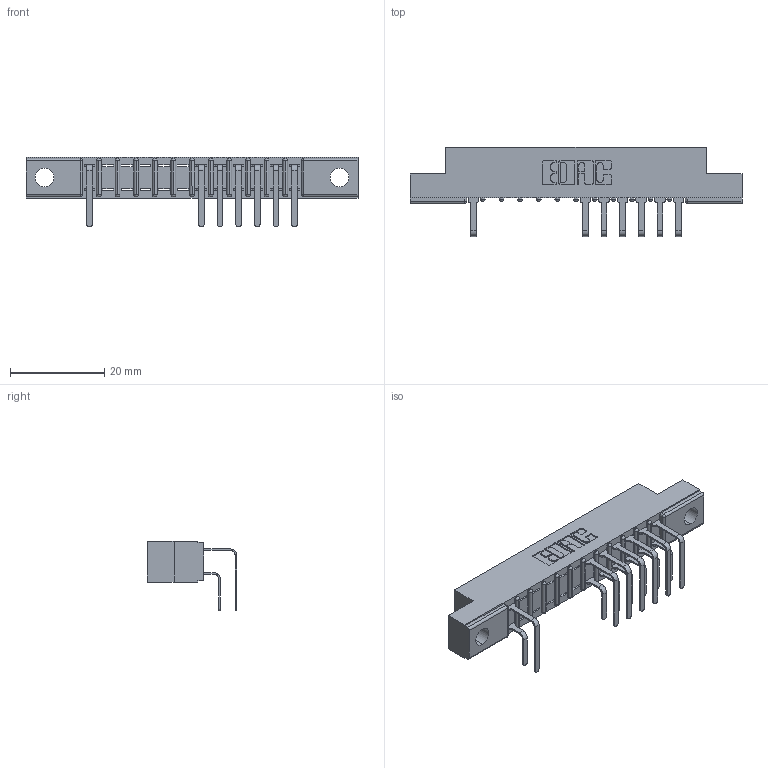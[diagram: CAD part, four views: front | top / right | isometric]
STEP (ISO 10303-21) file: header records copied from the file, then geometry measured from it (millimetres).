
FILE_DESCRIPTION (( 'STEP AP203' ), '1' );
FILE_NAME ('307-012-558-104.STEP', '2018-08-02T22:31:34', ( '' ), ( '' ), 'SwSTEP 2.0', 'SolidWorks 2016', '' );
FILE_SCHEMA (( 'CONFIG_CONTROL_DESIGN' ));
Length unit declared in the file: inch
Products named in the file (4): 307 Part_.156 Dia Mounting Holes; 307-290-001_558 559 - 1 (Single); 307-290-001_558 - 2 (Single); 307-012-558-104
Assembly tree (15 placements, depth 2):
  307-012-558-104
    307 Part_.156 Dia Mounting Holes
    307-290-001_558 559 - 1 (Single)  x7
    307-290-001_558 - 2 (Single)  x7
Bounding box: 70.56 x 18.96 x 14.81 mm (x, y, z)
Volume: 4443.2 mm3; surface area: 6799.6 mm2
Topology: 15 solids, 15 shells, 945 faces, 2667 edges, 1722 vertices
Faces by surface type: plane 606, cylinder 313, sphere 26
Entity records: 15915 total; most frequent: CARTESIAN_POINT 2662, ORIENTED_EDGE 2642, DIRECTION 2601, EDGE_CURVE 1321, VECTOR 1007, LINE 1007, VERTEX_POINT 858, AXIS2_PLACEMENT_3D 797
